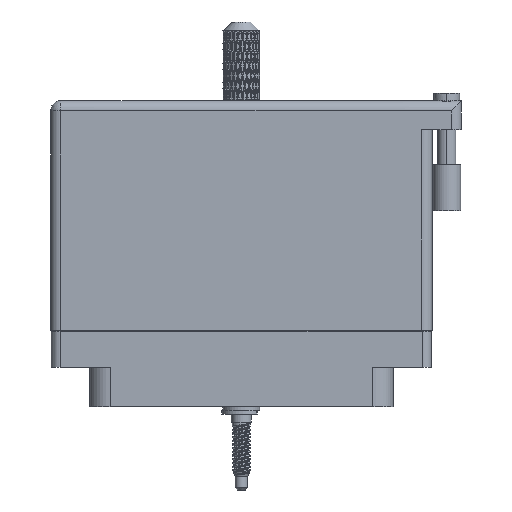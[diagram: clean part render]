
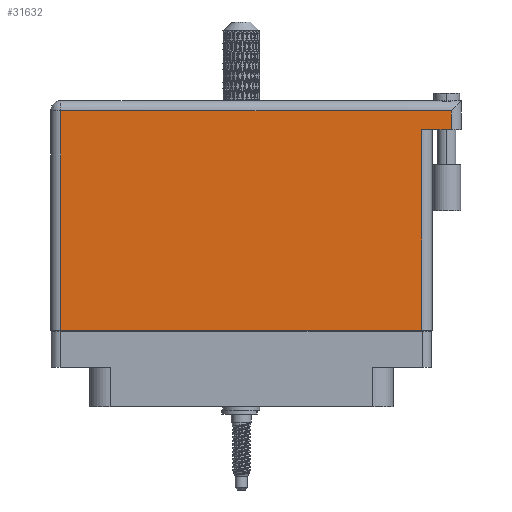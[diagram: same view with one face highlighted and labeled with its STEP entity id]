
A CAD part, front view. The second image highlights one B-rep face of the part: STEP entity #31632.
In plain terms, the highlighted face is planar.
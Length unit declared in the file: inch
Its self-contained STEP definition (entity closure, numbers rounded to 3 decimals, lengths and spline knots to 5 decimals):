
#2781 = ORIENTED_EDGE ( 'NONE', *, *, #71061, .T. ) ;
#3197 = VECTOR ( 'NONE', #25013, 39.37008 ) ;
#3903 = CARTESIAN_POINT ( 'NONE',  ( -1.3, 1.466, 0.4495 ) ) ;
#4301 = DIRECTION ( 'NONE',  ( 0., 0., -1. ) ) ;
#5245 = DIRECTION ( 'NONE',  ( -1., 0., 0. ) ) ;
#8839 = CARTESIAN_POINT ( 'NONE',  ( -1.23, -0.1, 0.4495 ) ) ;
#10760 = VERTEX_POINT ( 'NONE', #74140 ) ;
#11511 = CARTESIAN_POINT ( 'NONE',  ( 1.5, 1.269, 0.4495 ) ) ;
#15888 = DIRECTION ( 'NONE',  ( 0., 1., 0. ) ) ;
#19274 = VECTOR ( 'NONE', #92522, 39.37008 ) ;
#19447 = DIRECTION ( 'NONE',  ( 1., 0., 0. ) ) ;
#22505 = PLANE ( 'NONE',  #90562 ) ;
#24270 = VECTOR ( 'NONE', #5245, 39.37008 ) ;
#25013 = DIRECTION ( 'NONE',  ( 0., 1., 0. ) ) ;
#25502 = EDGE_LOOP ( 'NONE', ( #39884, #67015, #31291, #52697, #2781, #38755 ) ) ;
#27634 = CARTESIAN_POINT ( 'NONE',  ( 1.23, 1.269, 0.4495 ) ) ;
#29291 = DIRECTION ( 'NONE',  ( -1., 0., 0. ) ) ;
#31291 = ORIENTED_EDGE ( 'NONE', *, *, #57830, .F. ) ;
#31567 = DIRECTION ( 'NONE',  ( -1., 0., 0. ) ) ;
#31632 = ADVANCED_FACE ( 'NONE', ( #83040 ), #22505, .F. ) ;
#32165 = CARTESIAN_POINT ( 'NONE',  ( 1.43, 1.269, 0.4495 ) ) ;
#37605 = CARTESIAN_POINT ( 'NONE',  ( -1.23, -0.1, 0.4495 ) ) ;
#38755 = ORIENTED_EDGE ( 'NONE', *, *, #62630, .T. ) ;
#39884 = ORIENTED_EDGE ( 'NONE', *, *, #112538, .T. ) ;
#42364 = VERTEX_POINT ( 'NONE', #32165 ) ;
#43362 = CARTESIAN_POINT ( 'NONE',  ( 1.43, 1.396, 0.4495 ) ) ;
#44271 = LINE ( 'NONE', #79243, #3197 ) ;
#52697 = ORIENTED_EDGE ( 'NONE', *, *, #106866, .T. ) ;
#56257 = CARTESIAN_POINT ( 'NONE',  ( -1.3, -0.1, 0.4495 ) ) ;
#57470 = VECTOR ( 'NONE', #15888, 39.37008 ) ;
#57830 = EDGE_CURVE ( 'NONE', #42364, #112835, #105363, .T. ) ;
#58568 = VERTEX_POINT ( 'NONE', #43362 ) ;
#60915 = VERTEX_POINT ( 'NONE', #8839 ) ;
#62630 = EDGE_CURVE ( 'NONE', #10760, #60915, #108576, .T. ) ;
#63116 = LINE ( 'NONE', #106499, #57470 ) ;
#67015 = ORIENTED_EDGE ( 'NONE', *, *, #110498, .T. ) ;
#69581 = LINE ( 'NONE', #96581, #24270 ) ;
#71061 = EDGE_CURVE ( 'NONE', #58568, #10760, #69581, .T. ) ;
#73762 = LINE ( 'NONE', #56257, #97832 ) ;
#74140 = CARTESIAN_POINT ( 'NONE',  ( -1.23, 1.396, 0.4495 ) ) ;
#77816 = CARTESIAN_POINT ( 'NONE',  ( 1.23, -0.1, 0.4495 ) ) ;
#79243 = CARTESIAN_POINT ( 'NONE',  ( 1.23, 1.269, 0.4495 ) ) ;
#83040 = FACE_OUTER_BOUND ( 'NONE', #25502, .T. ) ;
#90562 = AXIS2_PLACEMENT_3D ( 'NONE', #3903, #4301, #31567 ) ;
#91135 = VECTOR ( 'NONE', #29291, 39.37008 ) ;
#92522 = DIRECTION ( 'NONE',  ( 0., -1., 0. ) ) ;
#96581 = CARTESIAN_POINT ( 'NONE',  ( -1.3, 1.396, 0.4495 ) ) ;
#97832 = VECTOR ( 'NONE', #19447, 39.37008 ) ;
#102476 = VERTEX_POINT ( 'NONE', #77816 ) ;
#105363 = LINE ( 'NONE', #11511, #91135 ) ;
#106499 = CARTESIAN_POINT ( 'NONE',  ( 1.43, 1.466, 0.4495 ) ) ;
#106866 = EDGE_CURVE ( 'NONE', #42364, #58568, #63116, .T. ) ;
#108576 = LINE ( 'NONE', #37605, #19274 ) ;
#110498 = EDGE_CURVE ( 'NONE', #102476, #112835, #44271, .T. ) ;
#112538 = EDGE_CURVE ( 'NONE', #60915, #102476, #73762, .T. ) ;
#112835 = VERTEX_POINT ( 'NONE', #27634 ) ;
